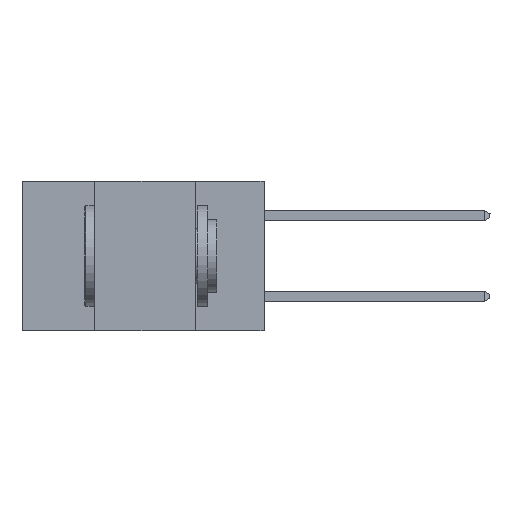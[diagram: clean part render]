
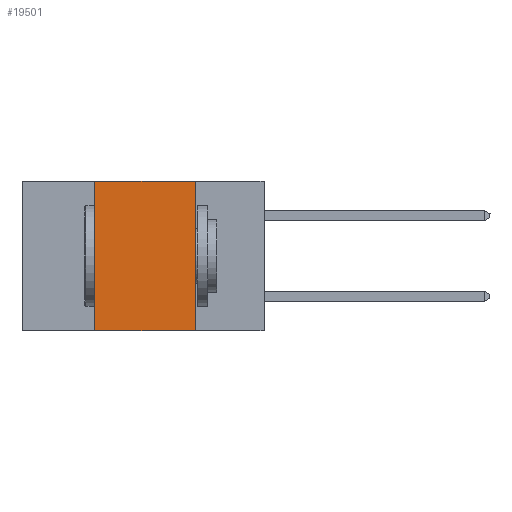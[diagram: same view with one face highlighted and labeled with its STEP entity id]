
A CAD part, left-side view. The second image highlights one B-rep face of the part: STEP entity #19501.
In plain terms, the highlighted planar face has unit normal (-1, 0, 0).
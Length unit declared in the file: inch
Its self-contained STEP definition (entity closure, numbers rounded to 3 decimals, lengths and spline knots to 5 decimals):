
#2825 = DIRECTION ( 'NONE',  ( 0., 0., 1. ) ) ;
#3955 = VERTEX_POINT ( 'NONE', #18146 ) ;
#4666 = VECTOR ( 'NONE', #4898, 39.37008 ) ;
#4898 = DIRECTION ( 'NONE',  ( 0., 0., -1. ) ) ;
#5369 = DIRECTION ( 'NONE',  ( 1., 0., 0. ) ) ;
#6214 = VECTOR ( 'NONE', #2825, 39.37008 ) ;
#7717 = ORIENTED_EDGE ( 'NONE', *, *, #13284, .T. ) ;
#8670 = CARTESIAN_POINT ( 'NONE',  ( 0., 0.42, -0.37 ) ) ;
#10178 = VECTOR ( 'NONE', #18319, 39.37008 ) ;
#11784 = ORIENTED_EDGE ( 'NONE', *, *, #24244, .F. ) ;
#12033 = LINE ( 'NONE', #22894, #6214 ) ;
#13284 = EDGE_CURVE ( 'NONE', #22805, #14707, #21209, .T. ) ;
#13451 = AXIS2_PLACEMENT_3D ( 'NONE', #20211, #5369, #27981 ) ;
#13661 = EDGE_CURVE ( 'NONE', #22805, #3955, #12033, .T. ) ;
#13822 = VECTOR ( 'NONE', #28243, 39.37008 ) ;
#14707 = VERTEX_POINT ( 'NONE', #18192 ) ;
#15797 = CARTESIAN_POINT ( 'NONE',  ( 0., 0.6, 0. ) ) ;
#17177 = EDGE_LOOP ( 'NONE', ( #11784, #24453, #17508, #7717 ) ) ;
#17508 = ORIENTED_EDGE ( 'NONE', *, *, #13661, .F. ) ;
#18146 = CARTESIAN_POINT ( 'NONE',  ( 0., 0.42, 0. ) ) ;
#18192 = CARTESIAN_POINT ( 'NONE',  ( 0., 0.17, -0.37 ) ) ;
#18319 = DIRECTION ( 'NONE',  ( 0., -1., 0. ) ) ;
#19317 = EDGE_CURVE ( 'NONE', #3955, #22932, #23760, .T. ) ;
#19501 = ADVANCED_FACE ( 'NONE', ( #19800 ), #27211, .F. ) ;
#19800 = FACE_OUTER_BOUND ( 'NONE', #17177, .T. ) ;
#20211 = CARTESIAN_POINT ( 'NONE',  ( 0., 0.6, 0. ) ) ;
#21209 = LINE ( 'NONE', #25793, #13822 ) ;
#22805 = VERTEX_POINT ( 'NONE', #8670 ) ;
#22894 = CARTESIAN_POINT ( 'NONE',  ( 0., 0.42, 0. ) ) ;
#22932 = VERTEX_POINT ( 'NONE', #31785 ) ;
#23760 = LINE ( 'NONE', #15797, #10178 ) ;
#24244 = EDGE_CURVE ( 'NONE', #22932, #14707, #31092, .T. ) ;
#24453 = ORIENTED_EDGE ( 'NONE', *, *, #19317, .F. ) ;
#25793 = CARTESIAN_POINT ( 'NONE',  ( 0., 0.6, -0.37 ) ) ;
#26882 = CARTESIAN_POINT ( 'NONE',  ( 0., 0.17, 0. ) ) ;
#27211 = PLANE ( 'NONE',  #13451 ) ;
#27981 = DIRECTION ( 'NONE',  ( 0., 0., -1. ) ) ;
#28243 = DIRECTION ( 'NONE',  ( 0., -1., 0. ) ) ;
#31092 = LINE ( 'NONE', #26882, #4666 ) ;
#31785 = CARTESIAN_POINT ( 'NONE',  ( 0., 0.17, 0. ) ) ;
